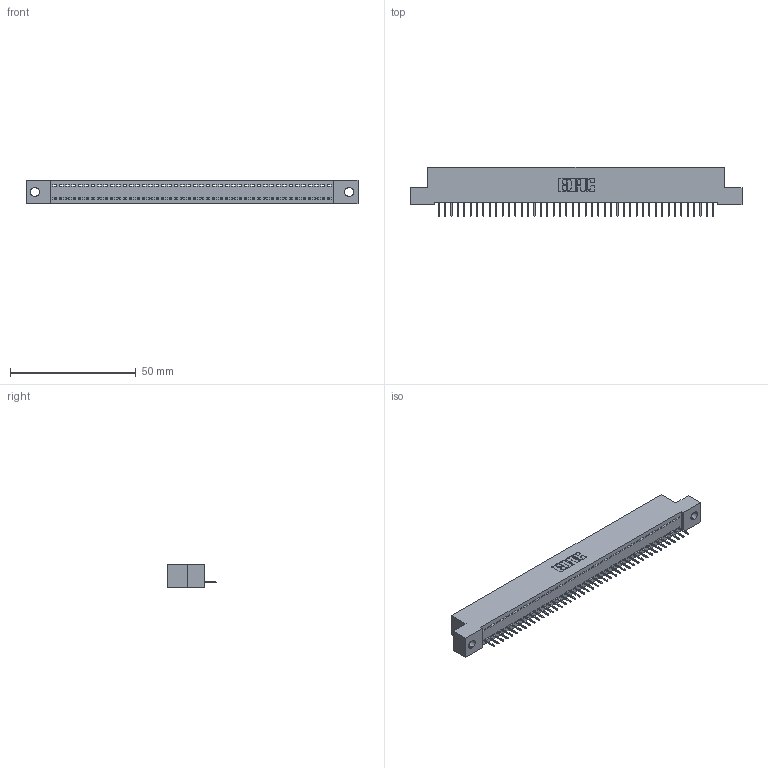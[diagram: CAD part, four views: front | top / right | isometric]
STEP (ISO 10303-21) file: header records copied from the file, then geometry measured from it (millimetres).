
FILE_DESCRIPTION (( 'STEP AP203' ), '1' );
FILE_NAME ('392-044-524-102.STEP', '2019-10-07T22:11:50', ( '' ), ( '' ), 'SwSTEP 2.0', 'SolidWorks 2016', '' );
FILE_SCHEMA (( 'CONFIG_CONTROL_DESIGN' ));
Length unit declared in the file: inch
Products named in the file (3): 342 Part_.128 Slot; 345-292-001_345-293-124; 392-044-524-102
Assembly tree (45 placements, depth 2):
  392-044-524-102
    342 Part_.128 Slot
    345-292-001_345-293-124  x44
Bounding box: 132.08 x 19.69 x 9.4 mm (x, y, z)
Volume: 11362.2 mm3; surface area: 15941.9 mm2
Topology: 45 solids, 45 shells, 2842 faces, 8231 edges, 5310 vertices
Faces by surface type: plane 2182, cylinder 660
Entity records: 26717 total; most frequent: CARTESIAN_POINT 4614, ORIENTED_EDGE 4594, DIRECTION 3889, EDGE_CURVE 2297, LINE 2173, VECTOR 2173, VERTEX_POINT 1526, AXIS2_PLACEMENT_3D 858
